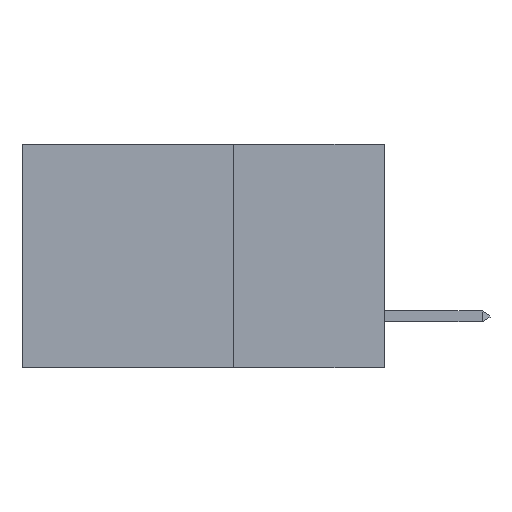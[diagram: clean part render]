
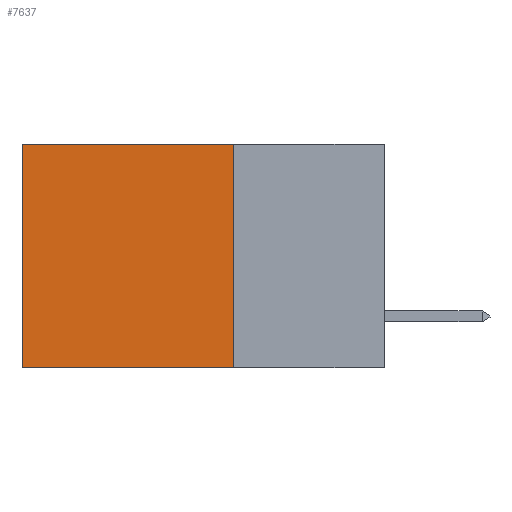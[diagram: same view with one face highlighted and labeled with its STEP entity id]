
A CAD part, left-side view. The second image highlights one B-rep face of the part: STEP entity #7637.
In plain terms, the highlighted planar face has unit normal (-1, 0, 0).
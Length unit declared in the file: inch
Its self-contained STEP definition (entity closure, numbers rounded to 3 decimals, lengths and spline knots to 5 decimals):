
#77 = CARTESIAN_POINT ( 'NONE',  ( 0.2875, 0.6, 0. ) ) ;
#460 = DIRECTION ( 'NONE',  ( 1., 0., 0. ) ) ;
#802 = CARTESIAN_POINT ( 'NONE',  ( 0.2875, 0.6, -0.37 ) ) ;
#1275 = LINE ( 'NONE', #6617, #5075 ) ;
#1616 = CARTESIAN_POINT ( 'NONE',  ( 0.2875, 0.25, -0.37 ) ) ;
#2011 = AXIS2_PLACEMENT_3D ( 'NONE', #6757, #460, #8934 ) ;
#2661 = CARTESIAN_POINT ( 'NONE',  ( 0.2875, 0.25, -0.37 ) ) ;
#2682 = ORIENTED_EDGE ( 'NONE', *, *, #11977, .T. ) ;
#2803 = ORIENTED_EDGE ( 'NONE', *, *, #8060, .F. ) ;
#2815 = ORIENTED_EDGE ( 'NONE', *, *, #8277, .F. ) ;
#2832 = ORIENTED_EDGE ( 'NONE', *, *, #6962, .T. ) ;
#2875 = LINE ( 'NONE', #8913, #8728 ) ;
#3958 = LINE ( 'NONE', #77, #7091 ) ;
#4830 = VERTEX_POINT ( 'NONE', #8477 ) ;
#4983 = EDGE_LOOP ( 'NONE', ( #2682, #2803, #2815, #2832 ) ) ;
#5075 = VECTOR ( 'NONE', #14172, 39.37008 ) ;
#5187 = VERTEX_POINT ( 'NONE', #5814 ) ;
#5814 = CARTESIAN_POINT ( 'NONE',  ( 0.2875, 0.6, 0. ) ) ;
#5993 = VECTOR ( 'NONE', #11740, 39.37008 ) ;
#6346 = LINE ( 'NONE', #2661, #5993 ) ;
#6617 = CARTESIAN_POINT ( 'NONE',  ( 0.2875, 0.25, 0. ) ) ;
#6757 = CARTESIAN_POINT ( 'NONE',  ( 0.2875, 0.25, 0. ) ) ;
#6962 = EDGE_CURVE ( 'NONE', #4830, #5187, #1275, .T. ) ;
#7091 = VECTOR ( 'NONE', #8638, 39.37008 ) ;
#7637 = ADVANCED_FACE ( 'NONE', ( #8576 ), #14302, .F. ) ;
#8060 = EDGE_CURVE ( 'NONE', #11006, #13531, #6346, .T. ) ;
#8277 = EDGE_CURVE ( 'NONE', #4830, #11006, #2875, .T. ) ;
#8477 = CARTESIAN_POINT ( 'NONE',  ( 0.2875, 0.25, 0. ) ) ;
#8576 = FACE_OUTER_BOUND ( 'NONE', #4983, .T. ) ;
#8638 = DIRECTION ( 'NONE',  ( 0., 0., -1. ) ) ;
#8728 = VECTOR ( 'NONE', #13191, 39.37008 ) ;
#8913 = CARTESIAN_POINT ( 'NONE',  ( 0.2875, 0.25, 0. ) ) ;
#8934 = DIRECTION ( 'NONE',  ( 0., 0., -1. ) ) ;
#11006 = VERTEX_POINT ( 'NONE', #1616 ) ;
#11740 = DIRECTION ( 'NONE',  ( 0., 1., 0. ) ) ;
#11977 = EDGE_CURVE ( 'NONE', #5187, #13531, #3958, .T. ) ;
#13191 = DIRECTION ( 'NONE',  ( 0., 0., -1. ) ) ;
#13531 = VERTEX_POINT ( 'NONE', #802 ) ;
#14172 = DIRECTION ( 'NONE',  ( 0., 1., 0. ) ) ;
#14302 = PLANE ( 'NONE',  #2011 ) ;
